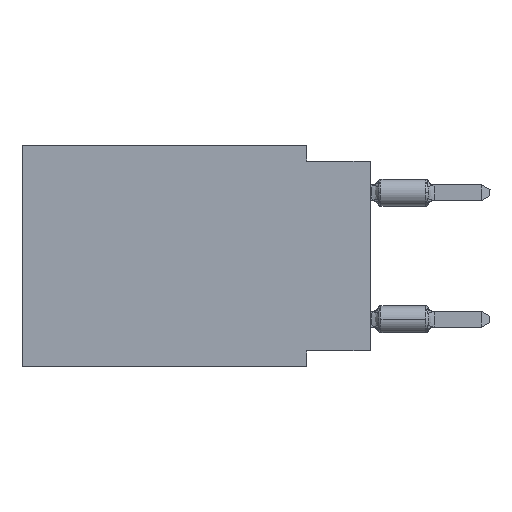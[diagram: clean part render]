
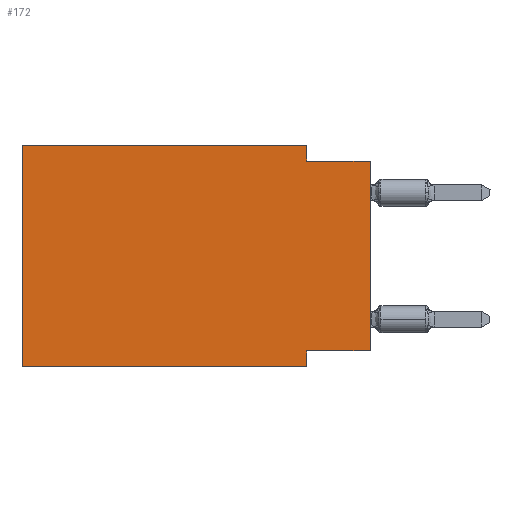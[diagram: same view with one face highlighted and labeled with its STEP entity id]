
A CAD part, left-side view. The second image highlights one B-rep face of the part: STEP entity #172.
In plain terms, the highlighted planar face has unit normal (-1, 0, 0).
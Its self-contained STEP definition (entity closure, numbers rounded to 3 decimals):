
#172 = ADVANCED_FACE ( 'NONE', ( #14881 ), #22482, .F. ) ;
#1427 = EDGE_CURVE ( 'NONE', #29850, #8665, #9059, .T. ) ;
#1608 = CARTESIAN_POINT ( 'NONE',  ( 0., 13.97, 0. ) ) ;
#2239 = ORIENTED_EDGE ( 'NONE', *, *, #16105, .F. ) ;
#2427 = EDGE_CURVE ( 'NONE', #33007, #16127, #33582, .T. ) ;
#2867 = ORIENTED_EDGE ( 'NONE', *, *, #10830, .T. ) ;
#4067 = ORIENTED_EDGE ( 'NONE', *, *, #27913, .F. ) ;
#4757 = EDGE_CURVE ( 'NONE', #8096, #29850, #6276, .T. ) ;
#5357 = EDGE_CURVE ( 'NONE', #18976, #33007, #17261, .T. ) ;
#5665 = ORIENTED_EDGE ( 'NONE', *, *, #4757, .F. ) ;
#6083 = VECTOR ( 'NONE', #27470, 1000. ) ;
#6276 = LINE ( 'NONE', #11105, #6083 ) ;
#7387 = DIRECTION ( 'NONE',  ( 0., -1., 0. ) ) ;
#8096 = VERTEX_POINT ( 'NONE', #20029 ) ;
#8665 = VERTEX_POINT ( 'NONE', #30698 ) ;
#9059 = LINE ( 'NONE', #14560, #15001 ) ;
#10517 = EDGE_LOOP ( 'NONE', ( #2867, #31714, #33304, #2239, #4067, #17114, #16403, #5665 ) ) ;
#10830 = EDGE_CURVE ( 'NONE', #8096, #16127, #16400, .T. ) ;
#11105 = CARTESIAN_POINT ( 'NONE',  ( 0., 0., -8.255 ) ) ;
#12444 = CARTESIAN_POINT ( 'NONE',  ( 0., 2.54, 0. ) ) ;
#13415 = VECTOR ( 'NONE', #7387, 1000. ) ;
#13858 = CARTESIAN_POINT ( 'NONE',  ( 0., 13.97, 0. ) ) ;
#13866 = LINE ( 'NONE', #24390, #33155 ) ;
#14033 = DIRECTION ( 'NONE',  ( 0., -1., 0. ) ) ;
#14447 = CARTESIAN_POINT ( 'NONE',  ( 0., 2.54, 0. ) ) ;
#14560 = CARTESIAN_POINT ( 'NONE',  ( 0., 2.54, -8.89 ) ) ;
#14881 = FACE_OUTER_BOUND ( 'NONE', #10517, .T. ) ;
#14952 = AXIS2_PLACEMENT_3D ( 'NONE', #1608, #27845, #24716 ) ;
#15001 = VECTOR ( 'NONE', #16444, 1000. ) ;
#15003 = CARTESIAN_POINT ( 'NONE',  ( 0., 13.97, 0. ) ) ;
#15530 = VECTOR ( 'NONE', #22942, 1000. ) ;
#16105 = EDGE_CURVE ( 'NONE', #20286, #18976, #20165, .T. ) ;
#16127 = VERTEX_POINT ( 'NONE', #25019 ) ;
#16400 = LINE ( 'NONE', #26429, #22006 ) ;
#16403 = ORIENTED_EDGE ( 'NONE', *, *, #1427, .F. ) ;
#16444 = DIRECTION ( 'NONE',  ( 0., 0., -1. ) ) ;
#17083 = VECTOR ( 'NONE', #27800, 1000. ) ;
#17114 = ORIENTED_EDGE ( 'NONE', *, *, #24552, .T. ) ;
#17261 = LINE ( 'NONE', #12444, #17083 ) ;
#18976 = VERTEX_POINT ( 'NONE', #14447 ) ;
#19150 = DIRECTION ( 'NONE',  ( 0., 0., 1. ) ) ;
#19491 = CARTESIAN_POINT ( 'NONE',  ( 0., 2.54, -8.255 ) ) ;
#19580 = CARTESIAN_POINT ( 'NONE',  ( 0., 2.54, -0.635 ) ) ;
#20029 = CARTESIAN_POINT ( 'NONE',  ( 0., 0., -8.255 ) ) ;
#20165 = LINE ( 'NONE', #15003, #15530 ) ;
#20286 = VERTEX_POINT ( 'NONE', #28065 ) ;
#22006 = VECTOR ( 'NONE', #19150, 1000. ) ;
#22482 = PLANE ( 'NONE',  #14952 ) ;
#22942 = DIRECTION ( 'NONE',  ( 0., -1., 0. ) ) ;
#23997 = CARTESIAN_POINT ( 'NONE',  ( 0., 13.97, -8.89 ) ) ;
#24385 = DIRECTION ( 'NONE',  ( 0., 0., 1. ) ) ;
#24390 = CARTESIAN_POINT ( 'NONE',  ( 0., 13.97, -8.89 ) ) ;
#24552 = EDGE_CURVE ( 'NONE', #30797, #8665, #13866, .T. ) ;
#24716 = DIRECTION ( 'NONE',  ( 0., 0., -1. ) ) ;
#25019 = CARTESIAN_POINT ( 'NONE',  ( 0., 0., -0.635 ) ) ;
#25600 = VECTOR ( 'NONE', #24385, 1000. ) ;
#26429 = CARTESIAN_POINT ( 'NONE',  ( 0., 0., 0. ) ) ;
#26971 = LINE ( 'NONE', #13858, #25600 ) ;
#27470 = DIRECTION ( 'NONE',  ( 0., 1., 0. ) ) ;
#27800 = DIRECTION ( 'NONE',  ( 0., 0., -1. ) ) ;
#27845 = DIRECTION ( 'NONE',  ( 1., 0., 0. ) ) ;
#27913 = EDGE_CURVE ( 'NONE', #30797, #20286, #26971, .T. ) ;
#28065 = CARTESIAN_POINT ( 'NONE',  ( 0., 13.97, 0. ) ) ;
#29850 = VERTEX_POINT ( 'NONE', #19491 ) ;
#30698 = CARTESIAN_POINT ( 'NONE',  ( 0., 2.54, -8.89 ) ) ;
#30797 = VERTEX_POINT ( 'NONE', #23997 ) ;
#31008 = CARTESIAN_POINT ( 'NONE',  ( 0., 0., -0.635 ) ) ;
#31714 = ORIENTED_EDGE ( 'NONE', *, *, #2427, .F. ) ;
#33007 = VERTEX_POINT ( 'NONE', #19580 ) ;
#33155 = VECTOR ( 'NONE', #14033, 1000. ) ;
#33304 = ORIENTED_EDGE ( 'NONE', *, *, #5357, .F. ) ;
#33582 = LINE ( 'NONE', #31008, #13415 ) ;
